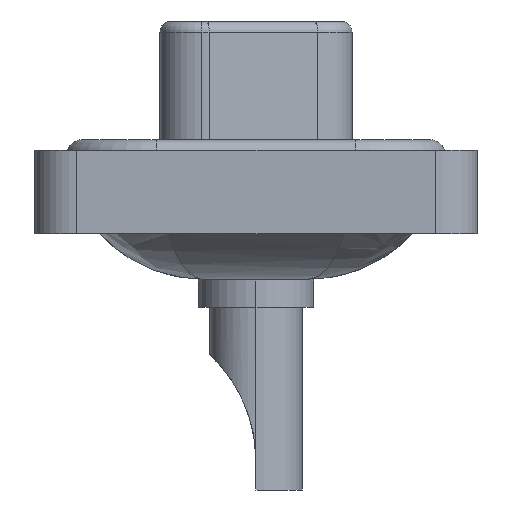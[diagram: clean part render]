
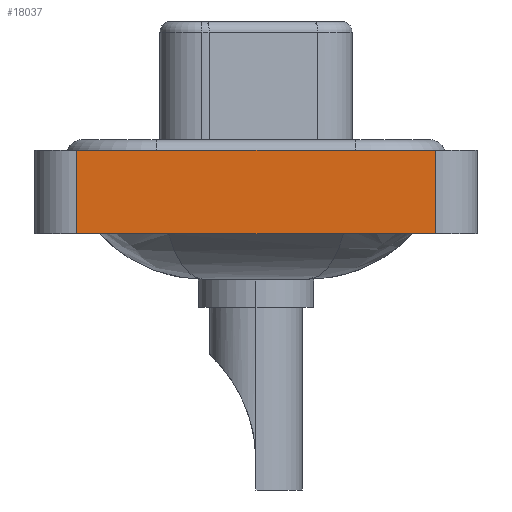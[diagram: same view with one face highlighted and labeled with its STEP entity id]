
A CAD part, left-side view. The second image highlights one B-rep face of the part: STEP entity #18037.
In plain terms, the highlighted planar face has unit normal (-1, 0, 0).
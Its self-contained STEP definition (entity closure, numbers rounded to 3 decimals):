
#499 = CARTESIAN_POINT ( 'NONE',  ( -7.35, 8.55, -3.6 ) ) ;
#1139 = VERTEX_POINT ( 'NONE', #19018 ) ;
#1976 = VECTOR ( 'NONE', #5423, 1000. ) ;
#2124 = ORIENTED_EDGE ( 'NONE', *, *, #5138, .F. ) ;
#3229 = VERTEX_POINT ( 'NONE', #12231 ) ;
#4211 = ORIENTED_EDGE ( 'NONE', *, *, #6760, .T. ) ;
#4404 = VECTOR ( 'NONE', #12432, 1000. ) ;
#4960 = EDGE_CURVE ( 'NONE', #22538, #3229, #20718, .T. ) ;
#5049 = LINE ( 'NONE', #20967, #5491 ) ;
#5138 = EDGE_CURVE ( 'NONE', #3229, #1139, #13769, .T. ) ;
#5423 = DIRECTION ( 'NONE',  ( 0., 0., 1. ) ) ;
#5491 = VECTOR ( 'NONE', #8413, 1000. ) ;
#6005 = DIRECTION ( 'NONE',  ( 0., 0., 1. ) ) ;
#6712 = CARTESIAN_POINT ( 'NONE',  ( -7.35, -8.55, 0.4 ) ) ;
#6760 = EDGE_CURVE ( 'NONE', #22538, #23024, #5049, .T. ) ;
#7481 = CARTESIAN_POINT ( 'NONE',  ( -7.35, 8.55, -3.6 ) ) ;
#8244 = EDGE_LOOP ( 'NONE', ( #10648, #2124, #15296, #4211 ) ) ;
#8413 = DIRECTION ( 'NONE',  ( 0., -1., 0. ) ) ;
#9293 = CARTESIAN_POINT ( 'NONE',  ( -7.35, -8.55, -3.6 ) ) ;
#10648 = ORIENTED_EDGE ( 'NONE', *, *, #15462, .T. ) ;
#12231 = CARTESIAN_POINT ( 'NONE',  ( -7.35, 8.55, 0.4 ) ) ;
#12432 = DIRECTION ( 'NONE',  ( 0., -1., 0. ) ) ;
#13769 = LINE ( 'NONE', #6712, #4404 ) ;
#14672 = PLANE ( 'NONE',  #17516 ) ;
#15296 = ORIENTED_EDGE ( 'NONE', *, *, #4960, .F. ) ;
#15462 = EDGE_CURVE ( 'NONE', #23024, #1139, #21661, .T. ) ;
#16354 = DIRECTION ( 'NONE',  ( 0., 0., 1. ) ) ;
#16589 = DIRECTION ( 'NONE',  ( -1., 0., 0. ) ) ;
#17516 = AXIS2_PLACEMENT_3D ( 'NONE', #9293, #16589, #16354 ) ;
#18037 = ADVANCED_FACE ( 'NONE', ( #18392 ), #14672, .T. ) ;
#18216 = CARTESIAN_POINT ( 'NONE',  ( -7.35, -8.55, -3.6 ) ) ;
#18392 = FACE_OUTER_BOUND ( 'NONE', #8244, .T. ) ;
#19018 = CARTESIAN_POINT ( 'NONE',  ( -7.35, -8.55, 0.4 ) ) ;
#19658 = VECTOR ( 'NONE', #6005, 1000. ) ;
#20718 = LINE ( 'NONE', #499, #19658 ) ;
#20967 = CARTESIAN_POINT ( 'NONE',  ( -7.35, -8.55, -3.6 ) ) ;
#21661 = LINE ( 'NONE', #18216, #1976 ) ;
#22538 = VERTEX_POINT ( 'NONE', #7481 ) ;
#23024 = VERTEX_POINT ( 'NONE', #23586 ) ;
#23586 = CARTESIAN_POINT ( 'NONE',  ( -7.35, -8.55, -3.6 ) ) ;
